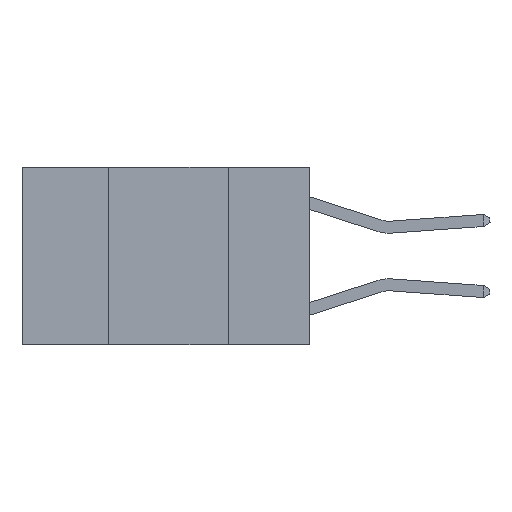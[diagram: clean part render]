
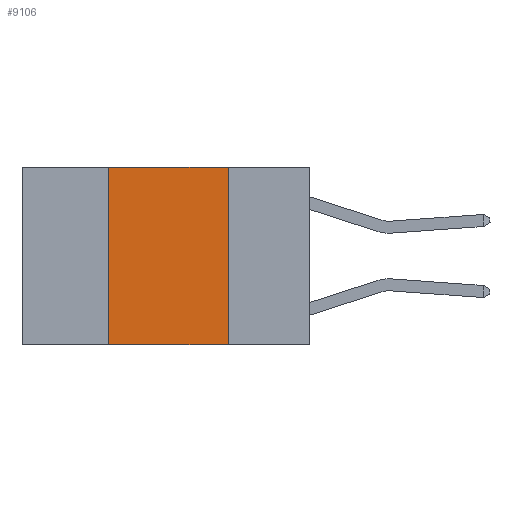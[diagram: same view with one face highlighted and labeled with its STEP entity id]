
A CAD part, left-side view. The second image highlights one B-rep face of the part: STEP entity #9106.
In plain terms, the highlighted planar face has unit normal (-1, 0, 0).
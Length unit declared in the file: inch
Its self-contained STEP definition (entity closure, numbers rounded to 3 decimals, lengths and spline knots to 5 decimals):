
#369 = LINE ( 'NONE', #7267, #1964 ) ;
#651 = DIRECTION ( 'NONE',  ( 1., 0., 0. ) ) ;
#962 = CARTESIAN_POINT ( 'NONE',  ( 0., 0.17, 0. ) ) ;
#1013 = DIRECTION ( 'NONE',  ( 0., 0., -1. ) ) ;
#1117 = CARTESIAN_POINT ( 'NONE',  ( 0., 0.42, -0.37 ) ) ;
#1323 = VERTEX_POINT ( 'NONE', #9051 ) ;
#1899 = EDGE_LOOP ( 'NONE', ( #2343, #7615, #2650, #4918 ) ) ;
#1964 = VECTOR ( 'NONE', #3738, 39.37008 ) ;
#2343 = ORIENTED_EDGE ( 'NONE', *, *, #8814, .F. ) ;
#2407 = AXIS2_PLACEMENT_3D ( 'NONE', #6914, #651, #9021 ) ;
#2524 = VECTOR ( 'NONE', #5066, 39.37008 ) ;
#2650 = ORIENTED_EDGE ( 'NONE', *, *, #4927, .F. ) ;
#2744 = EDGE_CURVE ( 'NONE', #8432, #1323, #369, .T. ) ;
#2858 = CARTESIAN_POINT ( 'NONE',  ( 0., 0.6, -0.37 ) ) ;
#2921 = FACE_OUTER_BOUND ( 'NONE', #1899, .T. ) ;
#2985 = LINE ( 'NONE', #9707, #2524 ) ;
#3378 = CARTESIAN_POINT ( 'NONE',  ( 0., 0.42, 0. ) ) ;
#3738 = DIRECTION ( 'NONE',  ( 0., -1., 0. ) ) ;
#4341 = DIRECTION ( 'NONE',  ( 0., -1., 0. ) ) ;
#4391 = LINE ( 'NONE', #2858, #8424 ) ;
#4635 = EDGE_CURVE ( 'NONE', #5280, #9040, #4391, .T. ) ;
#4764 = VECTOR ( 'NONE', #1013, 39.37008 ) ;
#4918 = ORIENTED_EDGE ( 'NONE', *, *, #4635, .T. ) ;
#4927 = EDGE_CURVE ( 'NONE', #5280, #8432, #2985, .T. ) ;
#5066 = DIRECTION ( 'NONE',  ( 0., 0., 1. ) ) ;
#5280 = VERTEX_POINT ( 'NONE', #1117 ) ;
#5512 = LINE ( 'NONE', #962, #4764 ) ;
#5955 = PLANE ( 'NONE',  #2407 ) ;
#6914 = CARTESIAN_POINT ( 'NONE',  ( 0., 0.6, 0. ) ) ;
#7267 = CARTESIAN_POINT ( 'NONE',  ( 0., 0.6, 0. ) ) ;
#7615 = ORIENTED_EDGE ( 'NONE', *, *, #2744, .F. ) ;
#8424 = VECTOR ( 'NONE', #4341, 39.37008 ) ;
#8432 = VERTEX_POINT ( 'NONE', #3378 ) ;
#8814 = EDGE_CURVE ( 'NONE', #1323, #9040, #5512, .T. ) ;
#9021 = DIRECTION ( 'NONE',  ( 0., 0., -1. ) ) ;
#9040 = VERTEX_POINT ( 'NONE', #9184 ) ;
#9051 = CARTESIAN_POINT ( 'NONE',  ( 0., 0.17, 0. ) ) ;
#9106 = ADVANCED_FACE ( 'NONE', ( #2921 ), #5955, .F. ) ;
#9184 = CARTESIAN_POINT ( 'NONE',  ( 0., 0.17, -0.37 ) ) ;
#9707 = CARTESIAN_POINT ( 'NONE',  ( 0., 0.42, 0. ) ) ;
